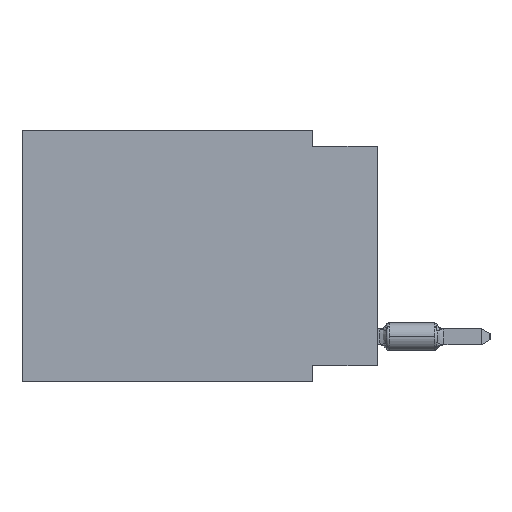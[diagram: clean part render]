
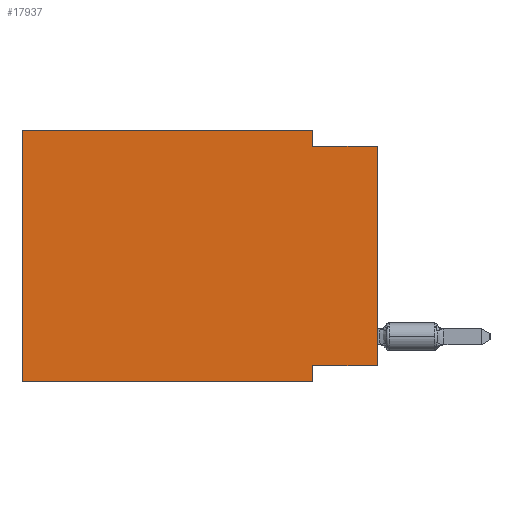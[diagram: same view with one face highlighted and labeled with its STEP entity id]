
A CAD part, left-side view. The second image highlights one B-rep face of the part: STEP entity #17937.
In plain terms, the highlighted planar face has unit normal (-1, 0, 0).
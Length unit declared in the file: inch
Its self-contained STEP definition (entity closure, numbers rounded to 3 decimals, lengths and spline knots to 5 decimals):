
#151 = VECTOR ( 'NONE', #7187, 39.37008 ) ;
#181 = VERTEX_POINT ( 'NONE', #900 ) ;
#381 = EDGE_CURVE ( 'NONE', #1544, #181, #5780, .T. ) ;
#900 = CARTESIAN_POINT ( 'NONE',  ( 0., 0.1, -0.025 ) ) ;
#1145 = VERTEX_POINT ( 'NONE', #8787 ) ;
#1544 = VERTEX_POINT ( 'NONE', #11910 ) ;
#1864 = CARTESIAN_POINT ( 'NONE',  ( 0., 0., -0.365 ) ) ;
#1922 = EDGE_CURVE ( 'NONE', #2754, #6707, #11473, .T. ) ;
#2233 = EDGE_CURVE ( 'NONE', #5944, #17857, #8685, .T. ) ;
#2424 = VERTEX_POINT ( 'NONE', #12043 ) ;
#2536 = ORIENTED_EDGE ( 'NONE', *, *, #18905, .T. ) ;
#2616 = ORIENTED_EDGE ( 'NONE', *, *, #381, .F. ) ;
#2703 = LINE ( 'NONE', #17889, #10617 ) ;
#2754 = VERTEX_POINT ( 'NONE', #6081 ) ;
#2787 = EDGE_CURVE ( 'NONE', #181, #1145, #2703, .T. ) ;
#3151 = VECTOR ( 'NONE', #4698, 39.37008 ) ;
#3260 = ORIENTED_EDGE ( 'NONE', *, *, #2787, .F. ) ;
#3694 = PLANE ( 'NONE',  #10441 ) ;
#4014 = LINE ( 'NONE', #17713, #13669 ) ;
#4296 = DIRECTION ( 'NONE',  ( 0., 0., -1. ) ) ;
#4297 = DIRECTION ( 'NONE',  ( 0., -1., 0. ) ) ;
#4698 = DIRECTION ( 'NONE',  ( 0., 0., 1. ) ) ;
#5043 = ORIENTED_EDGE ( 'NONE', *, *, #8613, .F. ) ;
#5187 = EDGE_CURVE ( 'NONE', #6707, #1544, #13210, .T. ) ;
#5293 = CARTESIAN_POINT ( 'NONE',  ( 0., 0.55, 0. ) ) ;
#5379 = DIRECTION ( 'NONE',  ( 1., 0., 0. ) ) ;
#5780 = LINE ( 'NONE', #17888, #18476 ) ;
#5944 = VERTEX_POINT ( 'NONE', #1864 ) ;
#6081 = CARTESIAN_POINT ( 'NONE',  ( 0., 0.55, -0.39 ) ) ;
#6203 = LINE ( 'NONE', #12235, #3151 ) ;
#6707 = VERTEX_POINT ( 'NONE', #8169 ) ;
#6731 = VECTOR ( 'NONE', #14732, 39.37008 ) ;
#7187 = DIRECTION ( 'NONE',  ( 0., -1., 0. ) ) ;
#7860 = ORIENTED_EDGE ( 'NONE', *, *, #1922, .F. ) ;
#8169 = CARTESIAN_POINT ( 'NONE',  ( 0., 0.55, 0. ) ) ;
#8371 = DIRECTION ( 'NONE',  ( 0., 0., -1. ) ) ;
#8613 = EDGE_CURVE ( 'NONE', #17857, #2424, #4014, .T. ) ;
#8685 = LINE ( 'NONE', #14623, #6731 ) ;
#8787 = CARTESIAN_POINT ( 'NONE',  ( 0., 0., -0.025 ) ) ;
#8791 = DIRECTION ( 'NONE',  ( 0., 0., -1. ) ) ;
#10003 = CARTESIAN_POINT ( 'NONE',  ( 0., 0.55, 0. ) ) ;
#10125 = ORIENTED_EDGE ( 'NONE', *, *, #11331, .T. ) ;
#10441 = AXIS2_PLACEMENT_3D ( 'NONE', #5293, #5379, #8371 ) ;
#10617 = VECTOR ( 'NONE', #4297, 39.37008 ) ;
#11331 = EDGE_CURVE ( 'NONE', #2754, #2424, #13019, .T. ) ;
#11384 = ORIENTED_EDGE ( 'NONE', *, *, #5187, .F. ) ;
#11473 = LINE ( 'NONE', #10003, #14604 ) ;
#11910 = CARTESIAN_POINT ( 'NONE',  ( 0., 0.1, 0. ) ) ;
#12043 = CARTESIAN_POINT ( 'NONE',  ( 0., 0.1, -0.39 ) ) ;
#12235 = CARTESIAN_POINT ( 'NONE',  ( 0., 0., 0. ) ) ;
#12632 = EDGE_LOOP ( 'NONE', ( #2536, #3260, #2616, #11384, #7860, #10125, #5043, #15921 ) ) ;
#12710 = FACE_OUTER_BOUND ( 'NONE', #12632, .T. ) ;
#13019 = LINE ( 'NONE', #19096, #14423 ) ;
#13210 = LINE ( 'NONE', #17690, #151 ) ;
#13669 = VECTOR ( 'NONE', #8791, 39.37008 ) ;
#14423 = VECTOR ( 'NONE', #17504, 39.37008 ) ;
#14604 = VECTOR ( 'NONE', #19033, 39.37008 ) ;
#14623 = CARTESIAN_POINT ( 'NONE',  ( 0., 0., -0.365 ) ) ;
#14732 = DIRECTION ( 'NONE',  ( 0., 1., 0. ) ) ;
#15921 = ORIENTED_EDGE ( 'NONE', *, *, #2233, .F. ) ;
#17504 = DIRECTION ( 'NONE',  ( 0., -1., 0. ) ) ;
#17690 = CARTESIAN_POINT ( 'NONE',  ( 0., 0.55, 0. ) ) ;
#17713 = CARTESIAN_POINT ( 'NONE',  ( 0., 0.1, -0.39 ) ) ;
#17857 = VERTEX_POINT ( 'NONE', #18692 ) ;
#17888 = CARTESIAN_POINT ( 'NONE',  ( 0., 0.1, 0. ) ) ;
#17889 = CARTESIAN_POINT ( 'NONE',  ( 0., 0., -0.025 ) ) ;
#17937 = ADVANCED_FACE ( 'NONE', ( #12710 ), #3694, .F. ) ;
#18476 = VECTOR ( 'NONE', #4296, 39.37008 ) ;
#18692 = CARTESIAN_POINT ( 'NONE',  ( 0., 0.1, -0.365 ) ) ;
#18905 = EDGE_CURVE ( 'NONE', #5944, #1145, #6203, .T. ) ;
#19033 = DIRECTION ( 'NONE',  ( 0., 0., 1. ) ) ;
#19096 = CARTESIAN_POINT ( 'NONE',  ( 0., 0.55, -0.39 ) ) ;
